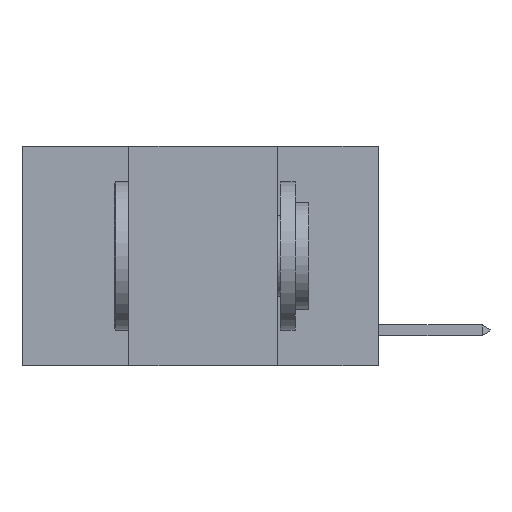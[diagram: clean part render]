
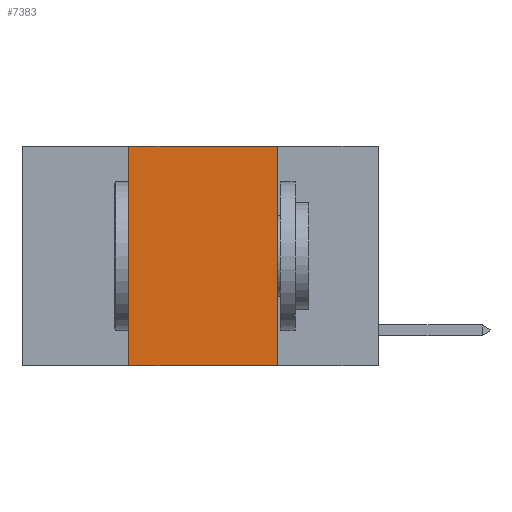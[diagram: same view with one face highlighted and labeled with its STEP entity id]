
A CAD part, left-side view. The second image highlights one B-rep face of the part: STEP entity #7383.
In plain terms, the highlighted planar face has unit normal (-1, 0, 0).
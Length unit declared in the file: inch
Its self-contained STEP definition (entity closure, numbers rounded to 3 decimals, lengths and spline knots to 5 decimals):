
#174 = CARTESIAN_POINT ( 'NONE',  ( 0., 0.17, -0.37 ) ) ;
#1485 = ORIENTED_EDGE ( 'NONE', *, *, #4885, .F. ) ;
#1608 = FACE_OUTER_BOUND ( 'NONE', #2394, .T. ) ;
#1865 = CARTESIAN_POINT ( 'NONE',  ( 0., 0.42, 0. ) ) ;
#2394 = EDGE_LOOP ( 'NONE', ( #18940, #1485, #11491, #12511 ) ) ;
#3613 = DIRECTION ( 'NONE',  ( 0., -1., 0. ) ) ;
#3764 = CARTESIAN_POINT ( 'NONE',  ( 0., 0.6, -0.37 ) ) ;
#3876 = CARTESIAN_POINT ( 'NONE',  ( 0., 0.17, 0. ) ) ;
#4851 = EDGE_CURVE ( 'NONE', #23304, #19680, #23801, .T. ) ;
#4885 = EDGE_CURVE ( 'NONE', #19680, #24031, #24718, .T. ) ;
#7142 = EDGE_CURVE ( 'NONE', #23304, #26981, #11013, .T. ) ;
#7383 = ADVANCED_FACE ( 'NONE', ( #1608 ), #19892, .F. ) ;
#8550 = VECTOR ( 'NONE', #26217, 39.37008 ) ;
#11013 = LINE ( 'NONE', #3764, #14457 ) ;
#11491 = ORIENTED_EDGE ( 'NONE', *, *, #4851, .F. ) ;
#12511 = ORIENTED_EDGE ( 'NONE', *, *, #7142, .T. ) ;
#12917 = VECTOR ( 'NONE', #12939, 39.37008 ) ;
#12939 = DIRECTION ( 'NONE',  ( 0., 0., -1. ) ) ;
#14377 = AXIS2_PLACEMENT_3D ( 'NONE', #26837, #15204, #17776 ) ;
#14457 = VECTOR ( 'NONE', #3613, 39.37008 ) ;
#15177 = CARTESIAN_POINT ( 'NONE',  ( 0., 0.6, 0. ) ) ;
#15204 = DIRECTION ( 'NONE',  ( 1., 0., 0. ) ) ;
#15527 = LINE ( 'NONE', #3876, #12917 ) ;
#17012 = CARTESIAN_POINT ( 'NONE',  ( 0., 0.42, 0. ) ) ;
#17776 = DIRECTION ( 'NONE',  ( 0., 0., -1. ) ) ;
#18940 = ORIENTED_EDGE ( 'NONE', *, *, #26476, .F. ) ;
#19680 = VERTEX_POINT ( 'NONE', #1865 ) ;
#19892 = PLANE ( 'NONE',  #14377 ) ;
#22563 = DIRECTION ( 'NONE',  ( 0., -1., 0. ) ) ;
#23304 = VERTEX_POINT ( 'NONE', #25731 ) ;
#23801 = LINE ( 'NONE', #17012, #8550 ) ;
#23918 = VECTOR ( 'NONE', #22563, 39.37008 ) ;
#24031 = VERTEX_POINT ( 'NONE', #25627 ) ;
#24718 = LINE ( 'NONE', #15177, #23918 ) ;
#25627 = CARTESIAN_POINT ( 'NONE',  ( 0., 0.17, 0. ) ) ;
#25731 = CARTESIAN_POINT ( 'NONE',  ( 0., 0.42, -0.37 ) ) ;
#26217 = DIRECTION ( 'NONE',  ( 0., 0., 1. ) ) ;
#26476 = EDGE_CURVE ( 'NONE', #24031, #26981, #15527, .T. ) ;
#26837 = CARTESIAN_POINT ( 'NONE',  ( 0., 0.6, 0. ) ) ;
#26981 = VERTEX_POINT ( 'NONE', #174 ) ;
